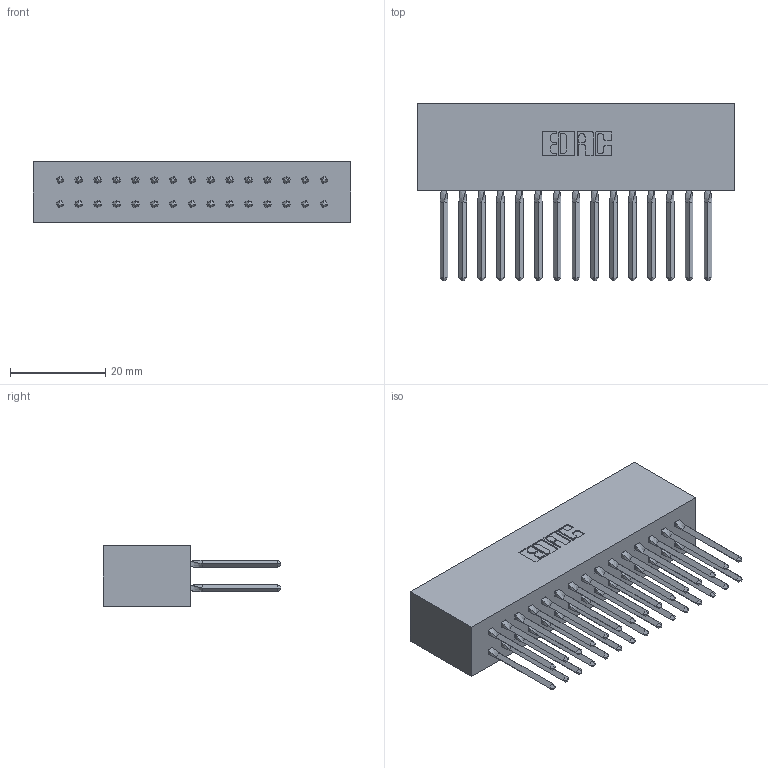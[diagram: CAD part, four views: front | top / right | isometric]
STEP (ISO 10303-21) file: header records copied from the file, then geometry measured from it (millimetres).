
FILE_DESCRIPTION (( 'STEP AP203' ), '1' );
FILE_NAME ('317-030-540-801.STEP', '2020-02-27T20:18:08', ( '' ), ( '' ), 'SwSTEP 2.0', 'SolidWorks 2016', '' );
FILE_SCHEMA (( 'CONFIG_CONTROL_DESIGN' ));
Length unit declared in the file: inch
Products named in the file (3): 317 Part_Lugless; 317-290-001_540; 317-030-540-801
Assembly tree (31 placements, depth 2):
  317-030-540-801
    317 Part_Lugless
    317-290-001_540  x30
Bounding box: 66.65 x 37.34 x 12.7 mm (x, y, z)
Volume: 12066.5 mm3; surface area: 17227 mm2
Topology: 31 solids, 31 shells, 2760 faces, 7649 edges, 4928 vertices
Faces by surface type: plane 2240, cylinder 400, bspline 120
Entity records: 25040 total; most frequent: CARTESIAN_POINT 4779, ORIENTED_EDGE 4278, DIRECTION 3565, EDGE_CURVE 2139, VECTOR 1891, LINE 1891, VERTEX_POINT 1419, AXIS2_PLACEMENT_3D 837
